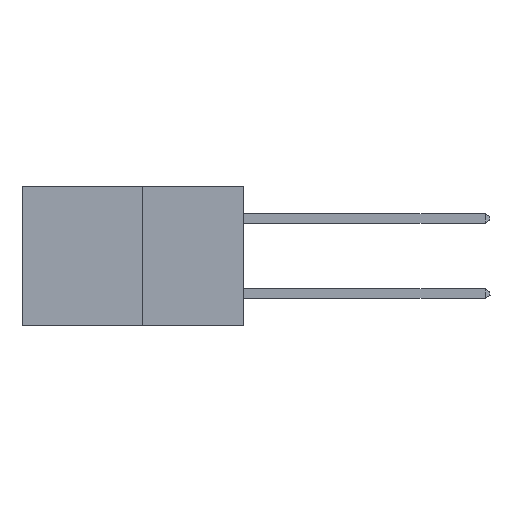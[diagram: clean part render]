
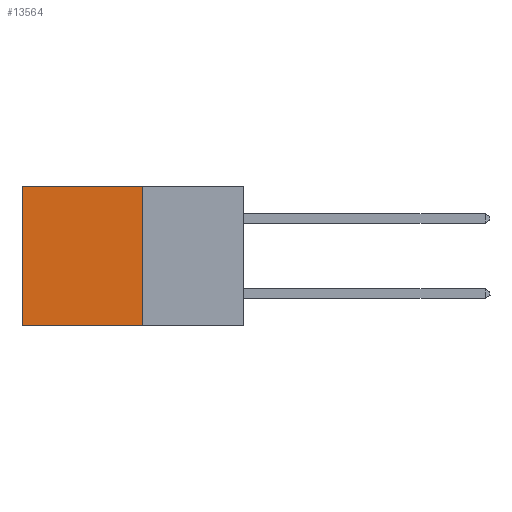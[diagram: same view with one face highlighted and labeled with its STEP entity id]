
A CAD part, left-side view. The second image highlights one B-rep face of the part: STEP entity #13564.
In plain terms, the highlighted planar face has unit normal (-1, 0, 0).
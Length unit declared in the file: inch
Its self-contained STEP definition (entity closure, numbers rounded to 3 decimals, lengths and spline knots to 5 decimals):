
#931 = ORIENTED_EDGE ( 'NONE', *, *, #8885, .T. ) ;
#948 = PLANE ( 'NONE',  #10049 ) ;
#2165 = CARTESIAN_POINT ( 'NONE',  ( 0.277, 0.27, -0.37 ) ) ;
#2281 = VERTEX_POINT ( 'NONE', #2165 ) ;
#2415 = CARTESIAN_POINT ( 'NONE',  ( 0.277, 0.27, -0.37 ) ) ;
#2780 = VERTEX_POINT ( 'NONE', #6619 ) ;
#3199 = FACE_OUTER_BOUND ( 'NONE', #13853, .T. ) ;
#3633 = EDGE_CURVE ( 'NONE', #2780, #2281, #11570, .T. ) ;
#3929 = ORIENTED_EDGE ( 'NONE', *, *, #8122, .F. ) ;
#4842 = CARTESIAN_POINT ( 'NONE',  ( 0.277, 0.59, 0. ) ) ;
#4892 = LINE ( 'NONE', #10605, #5273 ) ;
#5273 = VECTOR ( 'NONE', #5656, 39.37008 ) ;
#5656 = DIRECTION ( 'NONE',  ( 0., 1., 0. ) ) ;
#5946 = DIRECTION ( 'NONE',  ( 1., 0., 0. ) ) ;
#6619 = CARTESIAN_POINT ( 'NONE',  ( 0.277, 0.27, 0. ) ) ;
#7728 = CARTESIAN_POINT ( 'NONE',  ( 0.277, 0.59, -0.37 ) ) ;
#8082 = LINE ( 'NONE', #2415, #8838 ) ;
#8090 = VERTEX_POINT ( 'NONE', #4842 ) ;
#8122 = EDGE_CURVE ( 'NONE', #2281, #8607, #8082, .T. ) ;
#8607 = VERTEX_POINT ( 'NONE', #12078 ) ;
#8838 = VECTOR ( 'NONE', #9760, 39.37008 ) ;
#8885 = EDGE_CURVE ( 'NONE', #8090, #8607, #10736, .T. ) ;
#9587 = CARTESIAN_POINT ( 'NONE',  ( 0.277, 0.27, -0.37 ) ) ;
#9760 = DIRECTION ( 'NONE',  ( 0., 1., 0. ) ) ;
#10049 = AXIS2_PLACEMENT_3D ( 'NONE', #9587, #5946, #14442 ) ;
#10279 = ORIENTED_EDGE ( 'NONE', *, *, #14084, .T. ) ;
#10329 = VECTOR ( 'NONE', #14963, 39.37008 ) ;
#10605 = CARTESIAN_POINT ( 'NONE',  ( 0.277, 0.27, 0. ) ) ;
#10736 = LINE ( 'NONE', #7728, #10329 ) ;
#11194 = VECTOR ( 'NONE', #14362, 39.37008 ) ;
#11570 = LINE ( 'NONE', #12501, #11194 ) ;
#11846 = ORIENTED_EDGE ( 'NONE', *, *, #3633, .F. ) ;
#12078 = CARTESIAN_POINT ( 'NONE',  ( 0.277, 0.59, -0.37 ) ) ;
#12501 = CARTESIAN_POINT ( 'NONE',  ( 0.277, 0.27, -0.37 ) ) ;
#13564 = ADVANCED_FACE ( 'NONE', ( #3199 ), #948, .F. ) ;
#13853 = EDGE_LOOP ( 'NONE', ( #931, #3929, #11846, #10279 ) ) ;
#14084 = EDGE_CURVE ( 'NONE', #2780, #8090, #4892, .T. ) ;
#14362 = DIRECTION ( 'NONE',  ( 0., 0., -1. ) ) ;
#14442 = DIRECTION ( 'NONE',  ( 0., 0., -1. ) ) ;
#14963 = DIRECTION ( 'NONE',  ( 0., 0., -1. ) ) ;
